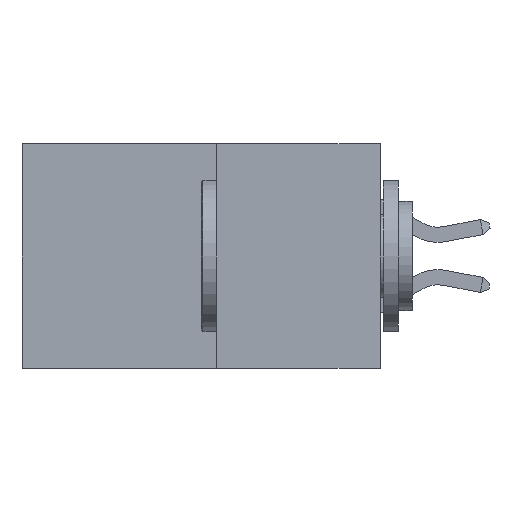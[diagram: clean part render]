
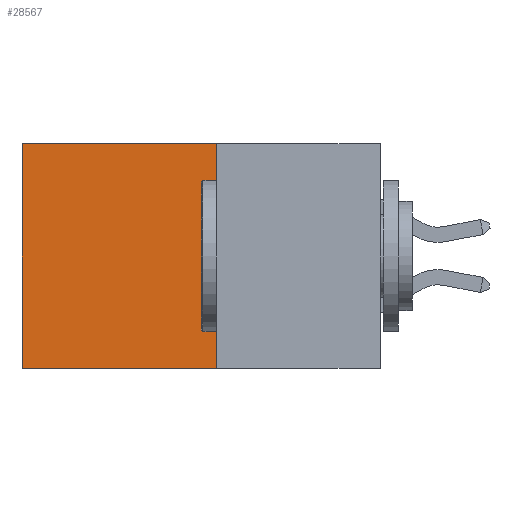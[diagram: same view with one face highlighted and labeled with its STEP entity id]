
A CAD part, left-side view. The second image highlights one B-rep face of the part: STEP entity #28567.
In plain terms, the highlighted planar face has unit normal (-1, 0, 0).
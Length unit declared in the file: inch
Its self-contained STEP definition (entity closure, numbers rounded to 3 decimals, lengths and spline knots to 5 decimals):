
#16 = LINE ( 'NONE', #28337, #5739 ) ;
#509 = EDGE_LOOP ( 'NONE', ( #1288, #23077, #16163, #29174 ) ) ;
#679 = VECTOR ( 'NONE', #16949, 39.37008 ) ;
#1288 = ORIENTED_EDGE ( 'NONE', *, *, #4592, .T. ) ;
#2829 = EDGE_CURVE ( 'NONE', #25694, #15540, #16, .T. ) ;
#3286 = CARTESIAN_POINT ( 'NONE',  ( 0.277, 0.27, -0.37 ) ) ;
#4592 = EDGE_CURVE ( 'NONE', #15540, #5915, #21664, .T. ) ;
#4661 = CARTESIAN_POINT ( 'NONE',  ( 0.277, 0.27, -0.37 ) ) ;
#5526 = DIRECTION ( 'NONE',  ( 0., 1., 0. ) ) ;
#5721 = DIRECTION ( 'NONE',  ( 0., 0., -1. ) ) ;
#5739 = VECTOR ( 'NONE', #6688, 39.37008 ) ;
#5915 = VERTEX_POINT ( 'NONE', #21959 ) ;
#6688 = DIRECTION ( 'NONE',  ( 0., 1., 0. ) ) ;
#8175 = LINE ( 'NONE', #28568, #26780 ) ;
#10116 = VERTEX_POINT ( 'NONE', #4661 ) ;
#11752 = CARTESIAN_POINT ( 'NONE',  ( 0.277, 0.59, 0. ) ) ;
#12498 = VECTOR ( 'NONE', #5526, 39.37008 ) ;
#13685 = AXIS2_PLACEMENT_3D ( 'NONE', #3286, #20360, #5721 ) ;
#15540 = VERTEX_POINT ( 'NONE', #11752 ) ;
#16163 = ORIENTED_EDGE ( 'NONE', *, *, #18939, .F. ) ;
#16949 = DIRECTION ( 'NONE',  ( 0., 0., -1. ) ) ;
#17293 = EDGE_CURVE ( 'NONE', #10116, #5915, #25373, .T. ) ;
#17934 = PLANE ( 'NONE',  #13685 ) ;
#18939 = EDGE_CURVE ( 'NONE', #25694, #10116, #8175, .T. ) ;
#19168 = CARTESIAN_POINT ( 'NONE',  ( 0.277, 0.59, -0.37 ) ) ;
#20360 = DIRECTION ( 'NONE',  ( 1., 0., 0. ) ) ;
#21664 = LINE ( 'NONE', #19168, #679 ) ;
#21959 = CARTESIAN_POINT ( 'NONE',  ( 0.277, 0.59, -0.37 ) ) ;
#23077 = ORIENTED_EDGE ( 'NONE', *, *, #17293, .F. ) ;
#25007 = CARTESIAN_POINT ( 'NONE',  ( 0.277, 0.27, -0.37 ) ) ;
#25373 = LINE ( 'NONE', #25007, #12498 ) ;
#25694 = VERTEX_POINT ( 'NONE', #29078 ) ;
#26780 = VECTOR ( 'NONE', #30976, 39.37008 ) ;
#28337 = CARTESIAN_POINT ( 'NONE',  ( 0.277, 0.27, 0. ) ) ;
#28567 = ADVANCED_FACE ( 'NONE', ( #29926 ), #17934, .F. ) ;
#28568 = CARTESIAN_POINT ( 'NONE',  ( 0.277, 0.27, -0.37 ) ) ;
#29078 = CARTESIAN_POINT ( 'NONE',  ( 0.277, 0.27, 0. ) ) ;
#29174 = ORIENTED_EDGE ( 'NONE', *, *, #2829, .T. ) ;
#29926 = FACE_OUTER_BOUND ( 'NONE', #509, .T. ) ;
#30976 = DIRECTION ( 'NONE',  ( 0., 0., -1. ) ) ;
